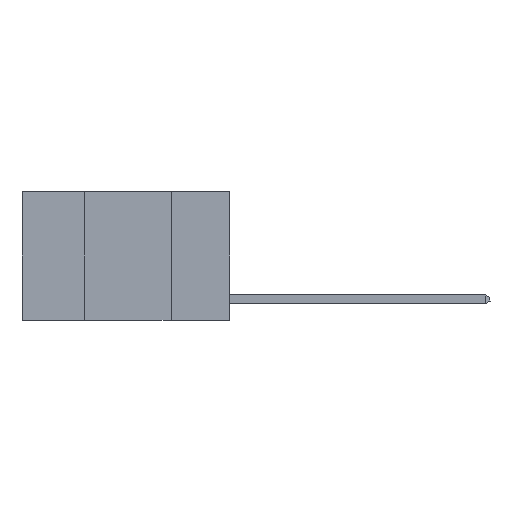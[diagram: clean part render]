
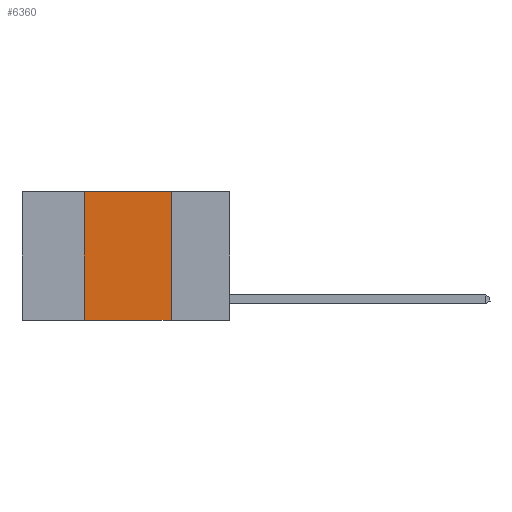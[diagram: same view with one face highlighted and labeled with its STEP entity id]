
A CAD part, left-side view. The second image highlights one B-rep face of the part: STEP entity #6360.
In plain terms, the highlighted planar face has unit normal (-1, 0, 0).
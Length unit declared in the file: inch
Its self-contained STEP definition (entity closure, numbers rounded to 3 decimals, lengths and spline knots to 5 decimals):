
#2595 = CARTESIAN_POINT ( 'NONE',  ( 0., 0.17, 0. ) ) ;
#3393 = CARTESIAN_POINT ( 'NONE',  ( 0., 0.42, -0.37 ) ) ;
#4103 = LINE ( 'NONE', #20846, #26704 ) ;
#4246 = CARTESIAN_POINT ( 'NONE',  ( 0., 0.6, 0. ) ) ;
#5213 = ORIENTED_EDGE ( 'NONE', *, *, #11157, .T. ) ;
#5841 = PLANE ( 'NONE',  #6989 ) ;
#6360 = ADVANCED_FACE ( 'NONE', ( #7034 ), #5841, .F. ) ;
#6498 = LINE ( 'NONE', #4246, #17440 ) ;
#6989 = AXIS2_PLACEMENT_3D ( 'NONE', #21153, #8015, #23364 ) ;
#7034 = FACE_OUTER_BOUND ( 'NONE', #14100, .T. ) ;
#8015 = DIRECTION ( 'NONE',  ( 1., 0., 0. ) ) ;
#9863 = VECTOR ( 'NONE', #15743, 39.37008 ) ;
#10033 = CARTESIAN_POINT ( 'NONE',  ( 0., 0.17, -0.37 ) ) ;
#11157 = EDGE_CURVE ( 'NONE', #23359, #13070, #4103, .T. ) ;
#13070 = VERTEX_POINT ( 'NONE', #10033 ) ;
#14078 = EDGE_CURVE ( 'NONE', #23359, #15545, #24076, .T. ) ;
#14100 = EDGE_LOOP ( 'NONE', ( #27758, #27707, #20894, #5213 ) ) ;
#15205 = VERTEX_POINT ( 'NONE', #2595 ) ;
#15545 = VERTEX_POINT ( 'NONE', #21151 ) ;
#15743 = DIRECTION ( 'NONE',  ( 0., 0., -1. ) ) ;
#17440 = VECTOR ( 'NONE', #23951, 39.37008 ) ;
#18141 = CARTESIAN_POINT ( 'NONE',  ( 0., 0.42, 0. ) ) ;
#18231 = VECTOR ( 'NONE', #20352, 39.37008 ) ;
#18725 = DIRECTION ( 'NONE',  ( 0., -1., 0. ) ) ;
#19247 = EDGE_CURVE ( 'NONE', #15545, #15205, #6498, .T. ) ;
#19947 = EDGE_CURVE ( 'NONE', #15205, #13070, #21526, .T. ) ;
#20052 = CARTESIAN_POINT ( 'NONE',  ( 0., 0.17, 0. ) ) ;
#20352 = DIRECTION ( 'NONE',  ( 0., 0., 1. ) ) ;
#20846 = CARTESIAN_POINT ( 'NONE',  ( 0., 0.6, -0.37 ) ) ;
#20894 = ORIENTED_EDGE ( 'NONE', *, *, #14078, .F. ) ;
#21151 = CARTESIAN_POINT ( 'NONE',  ( 0., 0.42, 0. ) ) ;
#21153 = CARTESIAN_POINT ( 'NONE',  ( 0., 0.6, 0. ) ) ;
#21526 = LINE ( 'NONE', #20052, #9863 ) ;
#23359 = VERTEX_POINT ( 'NONE', #3393 ) ;
#23364 = DIRECTION ( 'NONE',  ( 0., 0., -1. ) ) ;
#23951 = DIRECTION ( 'NONE',  ( 0., -1., 0. ) ) ;
#24076 = LINE ( 'NONE', #18141, #18231 ) ;
#26704 = VECTOR ( 'NONE', #18725, 39.37008 ) ;
#27707 = ORIENTED_EDGE ( 'NONE', *, *, #19247, .F. ) ;
#27758 = ORIENTED_EDGE ( 'NONE', *, *, #19947, .F. ) ;
